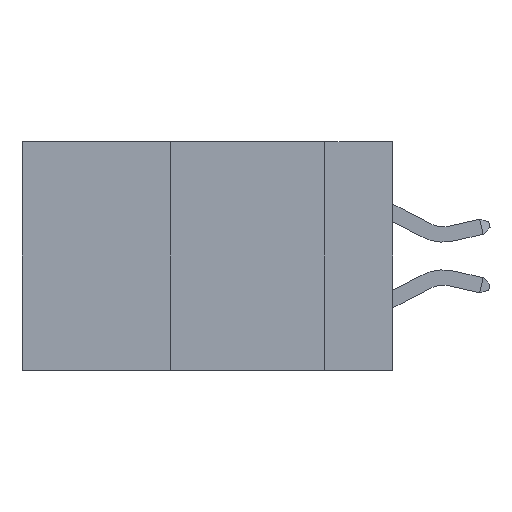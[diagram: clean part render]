
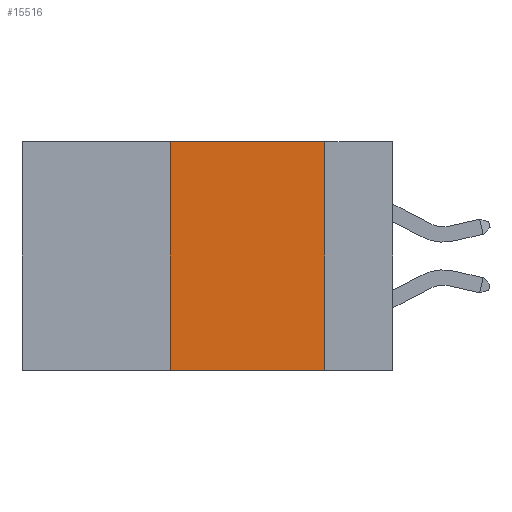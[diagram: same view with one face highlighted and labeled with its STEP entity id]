
A CAD part, left-side view. The second image highlights one B-rep face of the part: STEP entity #15516.
In plain terms, the highlighted planar face has unit normal (-1, 0, 0).
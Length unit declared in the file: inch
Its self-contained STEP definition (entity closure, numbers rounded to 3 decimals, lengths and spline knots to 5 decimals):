
#877 = AXIS2_PLACEMENT_3D ( 'NONE', #20783, #5949, #7466 ) ;
#2142 = VECTOR ( 'NONE', #16057, 39.37008 ) ;
#2301 = DIRECTION ( 'NONE',  ( 0., -1., 0. ) ) ;
#2485 = DIRECTION ( 'NONE',  ( 0., 0., -1. ) ) ;
#2569 = ORIENTED_EDGE ( 'NONE', *, *, #3021, .F. ) ;
#2672 = VECTOR ( 'NONE', #2485, 39.37008 ) ;
#2913 = VECTOR ( 'NONE', #2301, 39.37008 ) ;
#3021 = EDGE_CURVE ( 'NONE', #11089, #19598, #16158, .T. ) ;
#3919 = FACE_OUTER_BOUND ( 'NONE', #7223, .T. ) ;
#3921 = ORIENTED_EDGE ( 'NONE', *, *, #18321, .F. ) ;
#5556 = LINE ( 'NONE', #15616, #2913 ) ;
#5902 = ORIENTED_EDGE ( 'NONE', *, *, #9849, .F. ) ;
#5949 = DIRECTION ( 'NONE',  ( 1., 0., 0. ) ) ;
#7223 = EDGE_LOOP ( 'NONE', ( #3921, #5902, #2569, #9143 ) ) ;
#7466 = DIRECTION ( 'NONE',  ( 0., 0., -1. ) ) ;
#7632 = CARTESIAN_POINT ( 'NONE',  ( 0., 0.6, 0. ) ) ;
#8539 = VERTEX_POINT ( 'NONE', #15551 ) ;
#9143 = ORIENTED_EDGE ( 'NONE', *, *, #15091, .T. ) ;
#9356 = DIRECTION ( 'NONE',  ( 0., -1., 0. ) ) ;
#9849 = EDGE_CURVE ( 'NONE', #19598, #8539, #12517, .T. ) ;
#11089 = VERTEX_POINT ( 'NONE', #20633 ) ;
#12517 = LINE ( 'NONE', #7632, #12834 ) ;
#12834 = VECTOR ( 'NONE', #9356, 39.37008 ) ;
#14272 = LINE ( 'NONE', #20780, #2672 ) ;
#15091 = EDGE_CURVE ( 'NONE', #11089, #17634, #5556, .T. ) ;
#15516 = ADVANCED_FACE ( 'NONE', ( #3919 ), #20375, .F. ) ;
#15551 = CARTESIAN_POINT ( 'NONE',  ( 0., 0.11, 0. ) ) ;
#15616 = CARTESIAN_POINT ( 'NONE',  ( 0., 0.6, -0.37 ) ) ;
#16057 = DIRECTION ( 'NONE',  ( 0., 0., 1. ) ) ;
#16158 = LINE ( 'NONE', #20711, #2142 ) ;
#17634 = VERTEX_POINT ( 'NONE', #21056 ) ;
#18321 = EDGE_CURVE ( 'NONE', #8539, #17634, #14272, .T. ) ;
#19598 = VERTEX_POINT ( 'NONE', #19937 ) ;
#19937 = CARTESIAN_POINT ( 'NONE',  ( 0., 0.36, 0. ) ) ;
#20375 = PLANE ( 'NONE',  #877 ) ;
#20633 = CARTESIAN_POINT ( 'NONE',  ( 0., 0.36, -0.37 ) ) ;
#20711 = CARTESIAN_POINT ( 'NONE',  ( 0., 0.36, 0. ) ) ;
#20780 = CARTESIAN_POINT ( 'NONE',  ( 0., 0.11, 0. ) ) ;
#20783 = CARTESIAN_POINT ( 'NONE',  ( 0., 0.6, 0. ) ) ;
#21056 = CARTESIAN_POINT ( 'NONE',  ( 0., 0.11, -0.37 ) ) ;
